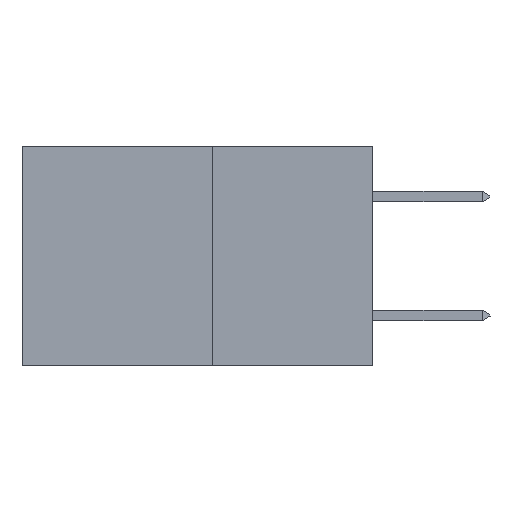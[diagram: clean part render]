
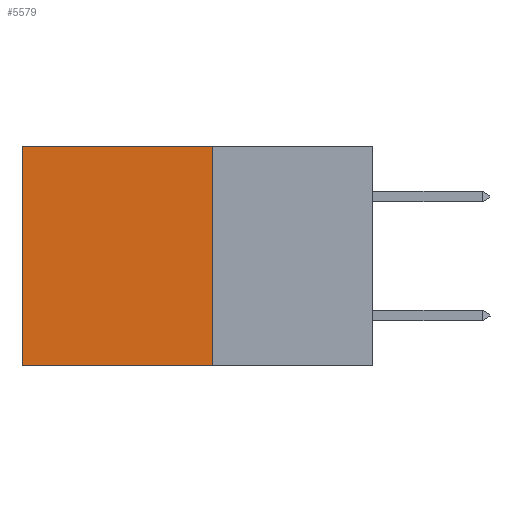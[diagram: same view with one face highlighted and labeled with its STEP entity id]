
A CAD part, left-side view. The second image highlights one B-rep face of the part: STEP entity #5579.
In plain terms, the highlighted planar face has unit normal (-1, 0, 0).
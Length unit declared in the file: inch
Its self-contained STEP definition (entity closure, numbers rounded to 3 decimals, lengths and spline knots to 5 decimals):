
#431 = DIRECTION ( 'NONE',  ( 0., 0., -1. ) ) ;
#1113 = VERTEX_POINT ( 'NONE', #6713 ) ;
#1286 = VERTEX_POINT ( 'NONE', #9473 ) ;
#1371 = PLANE ( 'NONE',  #4885 ) ;
#1480 = LINE ( 'NONE', #9378, #8604 ) ;
#1895 = ORIENTED_EDGE ( 'NONE', *, *, #4820, .T. ) ;
#2044 = ORIENTED_EDGE ( 'NONE', *, *, #8981, .F. ) ;
#2046 = DIRECTION ( 'NONE',  ( 0., 1., 0. ) ) ;
#2392 = ORIENTED_EDGE ( 'NONE', *, *, #3709, .T. ) ;
#2483 = ORIENTED_EDGE ( 'NONE', *, *, #3194, .F. ) ;
#3194 = EDGE_CURVE ( 'NONE', #6924, #1113, #5280, .T. ) ;
#3709 = EDGE_CURVE ( 'NONE', #6924, #6163, #8913, .T. ) ;
#3862 = EDGE_LOOP ( 'NONE', ( #1895, #2044, #2483, #2392 ) ) ;
#4251 = CARTESIAN_POINT ( 'NONE',  ( 0.277, 0.59, 0. ) ) ;
#4820 = EDGE_CURVE ( 'NONE', #6163, #1286, #1480, .T. ) ;
#4885 = AXIS2_PLACEMENT_3D ( 'NONE', #6284, #6255, #6180 ) ;
#5280 = LINE ( 'NONE', #8430, #8731 ) ;
#5579 = ADVANCED_FACE ( 'NONE', ( #8192 ), #1371, .F. ) ;
#5672 = LINE ( 'NONE', #5916, #9230 ) ;
#5916 = CARTESIAN_POINT ( 'NONE',  ( 0.277, 0.27, -0.37 ) ) ;
#6163 = VERTEX_POINT ( 'NONE', #4251 ) ;
#6180 = DIRECTION ( 'NONE',  ( 0., 0., -1. ) ) ;
#6255 = DIRECTION ( 'NONE',  ( 1., 0., 0. ) ) ;
#6284 = CARTESIAN_POINT ( 'NONE',  ( 0.277, 0.27, -0.37 ) ) ;
#6467 = CARTESIAN_POINT ( 'NONE',  ( 0.277, 0.27, 0. ) ) ;
#6713 = CARTESIAN_POINT ( 'NONE',  ( 0.277, 0.27, -0.37 ) ) ;
#6924 = VERTEX_POINT ( 'NONE', #6467 ) ;
#7307 = DIRECTION ( 'NONE',  ( 0., 1., 0. ) ) ;
#7371 = CARTESIAN_POINT ( 'NONE',  ( 0.277, 0.27, 0. ) ) ;
#8192 = FACE_OUTER_BOUND ( 'NONE', #3862, .T. ) ;
#8430 = CARTESIAN_POINT ( 'NONE',  ( 0.277, 0.27, -0.37 ) ) ;
#8604 = VECTOR ( 'NONE', #9281, 39.37008 ) ;
#8722 = VECTOR ( 'NONE', #7307, 39.37008 ) ;
#8731 = VECTOR ( 'NONE', #431, 39.37008 ) ;
#8913 = LINE ( 'NONE', #7371, #8722 ) ;
#8981 = EDGE_CURVE ( 'NONE', #1113, #1286, #5672, .T. ) ;
#9230 = VECTOR ( 'NONE', #2046, 39.37008 ) ;
#9281 = DIRECTION ( 'NONE',  ( 0., 0., -1. ) ) ;
#9378 = CARTESIAN_POINT ( 'NONE',  ( 0.277, 0.59, -0.37 ) ) ;
#9473 = CARTESIAN_POINT ( 'NONE',  ( 0.277, 0.59, -0.37 ) ) ;
